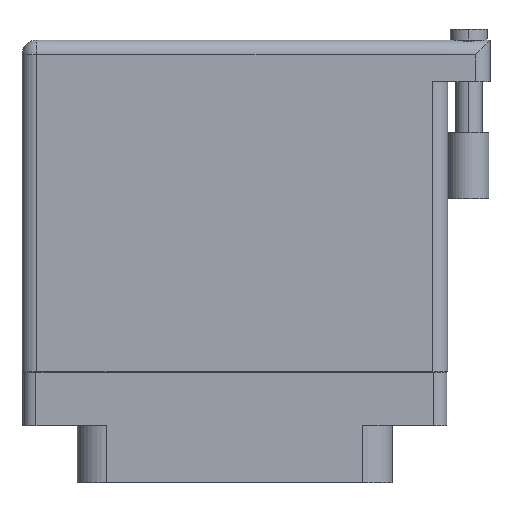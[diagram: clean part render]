
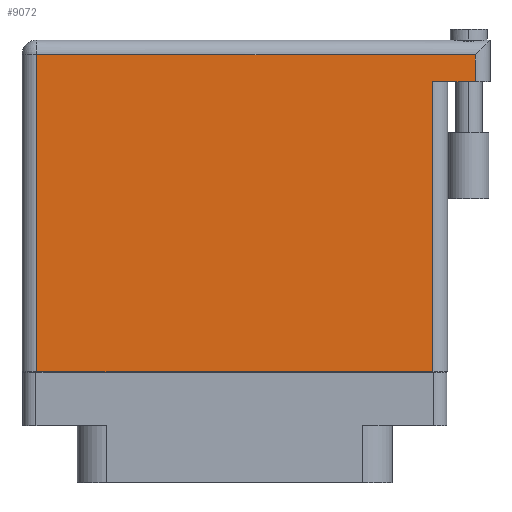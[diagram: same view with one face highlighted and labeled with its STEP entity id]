
A CAD part, front view. The second image highlights one B-rep face of the part: STEP entity #9072.
In plain terms, the highlighted face is planar.
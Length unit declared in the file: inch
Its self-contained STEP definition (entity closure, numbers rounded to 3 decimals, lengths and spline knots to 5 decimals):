
#460 = VERTEX_POINT ( 'NONE', #17514 ) ;
#928 = EDGE_CURVE ( 'NONE', #4363, #6343, #36560, .T. ) ;
#1152 = EDGE_CURVE ( 'NONE', #460, #11953, #10776, .T. ) ;
#1301 = VERTEX_POINT ( 'NONE', #27249 ) ;
#1594 = LINE ( 'NONE', #26758, #34378 ) ;
#1995 = EDGE_LOOP ( 'NONE', ( #7212, #12132, #15763, #26866, #34515, #3809 ) ) ;
#2005 = CARTESIAN_POINT ( 'NONE',  ( -1.004, 1.396, 0.4495 ) ) ;
#3390 = VECTOR ( 'NONE', #17716, 39.37008 ) ;
#3489 = EDGE_CURVE ( 'NONE', #6343, #1301, #5421, .T. ) ;
#3545 = VECTOR ( 'NONE', #24877, 39.37008 ) ;
#3809 = ORIENTED_EDGE ( 'NONE', *, *, #36503, .T. ) ;
#4113 = DIRECTION ( 'NONE',  ( 1., 0., 0. ) ) ;
#4363 = VERTEX_POINT ( 'NONE', #4384 ) ;
#4384 = CARTESIAN_POINT ( 'NONE',  ( 1.134, 1.269, 0.4495 ) ) ;
#5235 = EDGE_CURVE ( 'NONE', #11953, #35834, #16379, .T. ) ;
#5421 = LINE ( 'NONE', #2005, #3390 ) ;
#6088 = DIRECTION ( 'NONE',  ( 0., 0., -1. ) ) ;
#6343 = VERTEX_POINT ( 'NONE', #27806 ) ;
#7212 = ORIENTED_EDGE ( 'NONE', *, *, #1152, .T. ) ;
#9072 = ADVANCED_FACE ( 'NONE', ( #12129 ), #9108, .F. ) ;
#9108 = PLANE ( 'NONE',  #30226 ) ;
#10776 = LINE ( 'NONE', #23065, #19622 ) ;
#11953 = VERTEX_POINT ( 'NONE', #30419 ) ;
#12129 = FACE_OUTER_BOUND ( 'NONE', #1995, .T. ) ;
#12132 = ORIENTED_EDGE ( 'NONE', *, *, #5235, .T. ) ;
#15231 = CARTESIAN_POINT ( 'NONE',  ( 1.134, 1.466, 0.4495 ) ) ;
#15763 = ORIENTED_EDGE ( 'NONE', *, *, #20603, .F. ) ;
#16379 = LINE ( 'NONE', #22621, #35857 ) ;
#17514 = CARTESIAN_POINT ( 'NONE',  ( -0.934, -0.1, 0.4495 ) ) ;
#17716 = DIRECTION ( 'NONE',  ( -1., 0., 0. ) ) ;
#18417 = VECTOR ( 'NONE', #30318, 39.37008 ) ;
#19325 = LINE ( 'NONE', #24278, #3545 ) ;
#19622 = VECTOR ( 'NONE', #4113, 39.37008 ) ;
#20603 = EDGE_CURVE ( 'NONE', #4363, #35834, #1594, .T. ) ;
#22621 = CARTESIAN_POINT ( 'NONE',  ( 0.934, 1.269, 0.4495 ) ) ;
#23065 = CARTESIAN_POINT ( 'NONE',  ( -1.004, -0.1, 0.4495 ) ) ;
#23632 = CARTESIAN_POINT ( 'NONE',  ( 0.934, 1.269, 0.4495 ) ) ;
#24278 = CARTESIAN_POINT ( 'NONE',  ( -0.934, -0.1, 0.4495 ) ) ;
#24877 = DIRECTION ( 'NONE',  ( 0., -1., 0. ) ) ;
#26167 = DIRECTION ( 'NONE',  ( -1., 0., 0. ) ) ;
#26758 = CARTESIAN_POINT ( 'NONE',  ( 1.204, 1.269, 0.4495 ) ) ;
#26866 = ORIENTED_EDGE ( 'NONE', *, *, #928, .T. ) ;
#27249 = CARTESIAN_POINT ( 'NONE',  ( -0.934, 1.396, 0.4495 ) ) ;
#27806 = CARTESIAN_POINT ( 'NONE',  ( 1.134, 1.396, 0.4495 ) ) ;
#28220 = DIRECTION ( 'NONE',  ( -1., 0., 0. ) ) ;
#28246 = DIRECTION ( 'NONE',  ( 0., 1., 0. ) ) ;
#30226 = AXIS2_PLACEMENT_3D ( 'NONE', #33669, #6088, #28220 ) ;
#30318 = DIRECTION ( 'NONE',  ( 0., 1., 0. ) ) ;
#30419 = CARTESIAN_POINT ( 'NONE',  ( 0.934, -0.1, 0.4495 ) ) ;
#33669 = CARTESIAN_POINT ( 'NONE',  ( -1.004, 1.466, 0.4495 ) ) ;
#34378 = VECTOR ( 'NONE', #26167, 39.37008 ) ;
#34515 = ORIENTED_EDGE ( 'NONE', *, *, #3489, .T. ) ;
#35834 = VERTEX_POINT ( 'NONE', #23632 ) ;
#35857 = VECTOR ( 'NONE', #28246, 39.37008 ) ;
#36503 = EDGE_CURVE ( 'NONE', #1301, #460, #19325, .T. ) ;
#36560 = LINE ( 'NONE', #15231, #18417 ) ;
